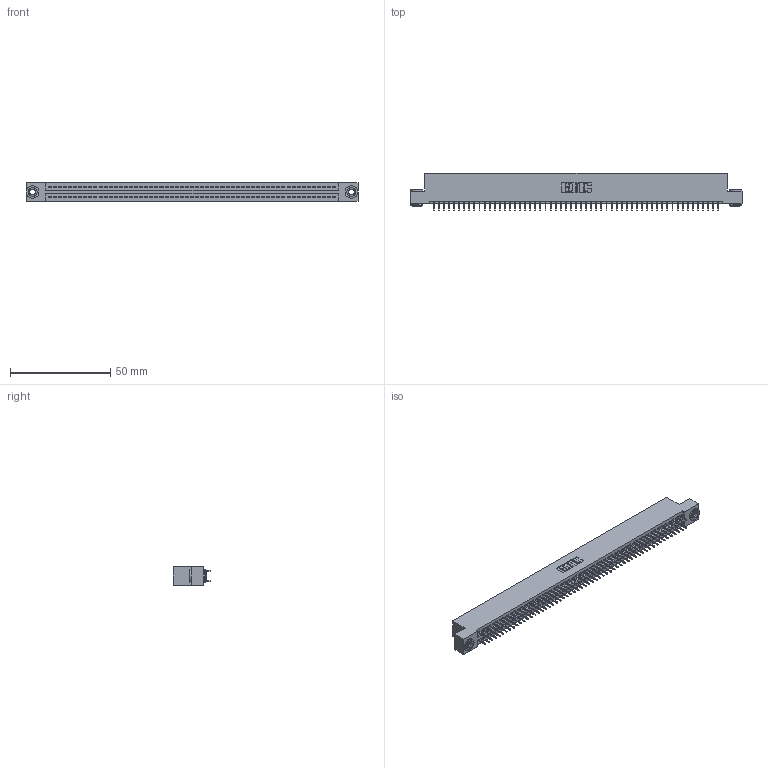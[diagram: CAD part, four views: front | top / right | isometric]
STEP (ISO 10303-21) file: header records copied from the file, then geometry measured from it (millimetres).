
FILE_DESCRIPTION (( 'STEP AP203' ), '1' );
FILE_NAME ('395-114-525-203.STEP', '2020-09-25T20:07:59', ( '' ), ( '' ), 'SwSTEP 2.0', 'SolidWorks 2020', '' );
FILE_SCHEMA (( 'CONFIG_CONTROL_DESIGN' ));
Length unit declared in the file: inch
Products named in the file (4): 345 Part_Flush Mounting Lugs - 0.156 Dia-TH; 395-114-525-203; 345-292-001_345-293-125; 345-250-002_345-250-002-102
Assembly tree (117 placements, depth 2):
  395-114-525-203
    345 Part_Flush Mounting Lugs - 0.156 Dia-TH
    345-292-001_345-293-125  x114
    345-250-002_345-250-002-102  x2
Bounding box: 165.99 x 18.72 x 9.4 mm (x, y, z)
Volume: 16095.3 mm3; surface area: 23721.6 mm2
Topology: 117 solids, 117 shells, 6320 faces, 17859 edges, 11446 vertices
Faces by surface type: plane 4536, cylinder 1776, cone 8
Entity records: 43428 total; most frequent: CARTESIAN_POINT 7239, ORIENTED_EDGE 7166, DIRECTION 6397, EDGE_CURVE 3583, LINE 3203, VECTOR 3203, VERTEX_POINT 2382, AXIS2_PLACEMENT_3D 1597
